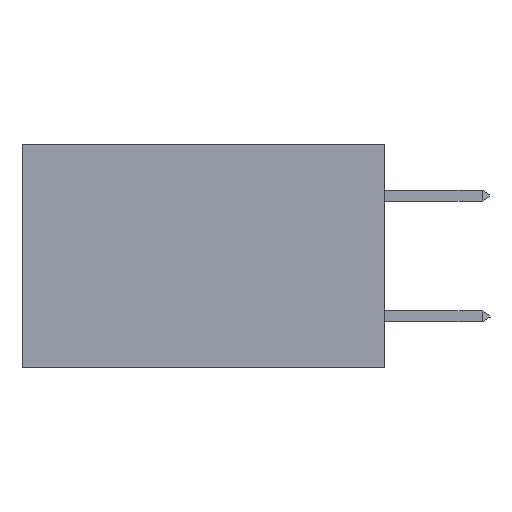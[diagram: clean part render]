
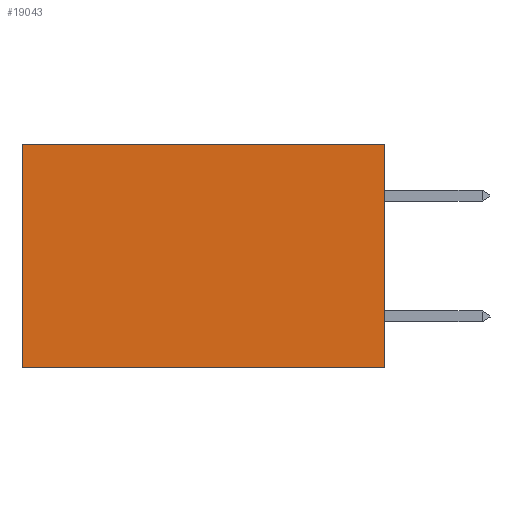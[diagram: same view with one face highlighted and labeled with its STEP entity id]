
A CAD part, left-side view. The second image highlights one B-rep face of the part: STEP entity #19043.
In plain terms, the highlighted planar face has unit normal (-1, 0, 0).
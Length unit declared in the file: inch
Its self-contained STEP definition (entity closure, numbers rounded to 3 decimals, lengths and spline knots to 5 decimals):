
#252 = ORIENTED_EDGE ( 'NONE', *, *, #32266, .T. ) ;
#2736 = VERTEX_POINT ( 'NONE', #18948 ) ;
#4488 = LINE ( 'NONE', #25973, #18414 ) ;
#5936 = VECTOR ( 'NONE', #32748, 39.37008 ) ;
#6471 = CARTESIAN_POINT ( 'NONE',  ( 0.2875, 0., -0.37 ) ) ;
#6925 = PLANE ( 'NONE',  #15320 ) ;
#7257 = CARTESIAN_POINT ( 'NONE',  ( 0.2875, 0.6, 0. ) ) ;
#7583 = FACE_OUTER_BOUND ( 'NONE', #33028, .T. ) ;
#8134 = VERTEX_POINT ( 'NONE', #7257 ) ;
#8838 = ORIENTED_EDGE ( 'NONE', *, *, #19374, .F. ) ;
#8879 = EDGE_CURVE ( 'NONE', #15733, #8134, #21827, .T. ) ;
#9268 = DIRECTION ( 'NONE',  ( 0., 1., 0. ) ) ;
#12535 = CARTESIAN_POINT ( 'NONE',  ( 0.2875, 0., 0. ) ) ;
#13091 = VECTOR ( 'NONE', #9268, 39.37008 ) ;
#13933 = LINE ( 'NONE', #6471, #13091 ) ;
#15291 = VECTOR ( 'NONE', #24089, 39.37008 ) ;
#15314 = DIRECTION ( 'NONE',  ( 0., 0., -1. ) ) ;
#15320 = AXIS2_PLACEMENT_3D ( 'NONE', #12535, #32019, #15314 ) ;
#15733 = VERTEX_POINT ( 'NONE', #20379 ) ;
#16866 = ORIENTED_EDGE ( 'NONE', *, *, #22001, .F. ) ;
#18414 = VECTOR ( 'NONE', #28776, 39.37008 ) ;
#18505 = CARTESIAN_POINT ( 'NONE',  ( 0.2875, 0., 0. ) ) ;
#18948 = CARTESIAN_POINT ( 'NONE',  ( 0.2875, 0., -0.37 ) ) ;
#19043 = ADVANCED_FACE ( 'NONE', ( #7583 ), #6925, .F. ) ;
#19374 = EDGE_CURVE ( 'NONE', #15733, #2736, #4488, .T. ) ;
#20379 = CARTESIAN_POINT ( 'NONE',  ( 0.2875, 0., 0. ) ) ;
#20566 = CARTESIAN_POINT ( 'NONE',  ( 0.2875, 0.6, -0.37 ) ) ;
#20746 = LINE ( 'NONE', #29907, #5936 ) ;
#21827 = LINE ( 'NONE', #18505, #15291 ) ;
#22001 = EDGE_CURVE ( 'NONE', #2736, #28775, #13933, .T. ) ;
#24089 = DIRECTION ( 'NONE',  ( 0., 1., 0. ) ) ;
#25973 = CARTESIAN_POINT ( 'NONE',  ( 0.2875, 0., 0. ) ) ;
#26799 = ORIENTED_EDGE ( 'NONE', *, *, #8879, .T. ) ;
#28775 = VERTEX_POINT ( 'NONE', #20566 ) ;
#28776 = DIRECTION ( 'NONE',  ( 0., 0., -1. ) ) ;
#29907 = CARTESIAN_POINT ( 'NONE',  ( 0.2875, 0.6, 0. ) ) ;
#32019 = DIRECTION ( 'NONE',  ( 1., 0., 0. ) ) ;
#32266 = EDGE_CURVE ( 'NONE', #8134, #28775, #20746, .T. ) ;
#32748 = DIRECTION ( 'NONE',  ( 0., 0., -1. ) ) ;
#33028 = EDGE_LOOP ( 'NONE', ( #252, #16866, #8838, #26799 ) ) ;
